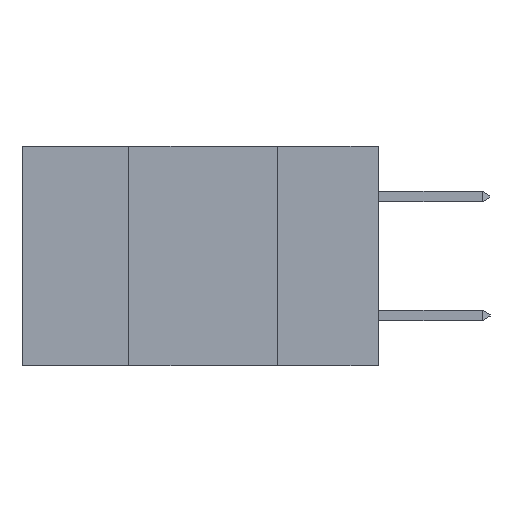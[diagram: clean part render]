
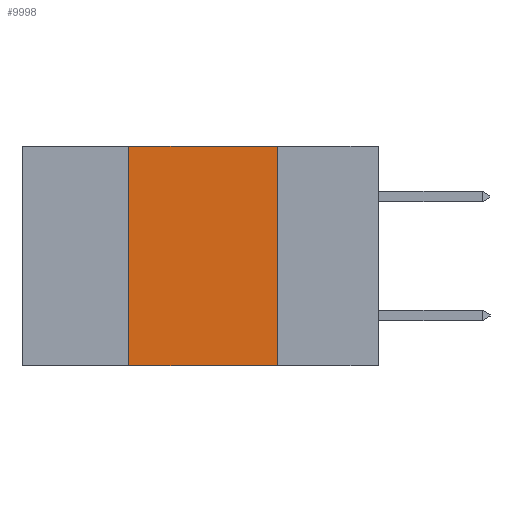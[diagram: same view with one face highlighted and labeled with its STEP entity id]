
A CAD part, left-side view. The second image highlights one B-rep face of the part: STEP entity #9998.
In plain terms, the highlighted planar face has unit normal (-1, 0, 0).
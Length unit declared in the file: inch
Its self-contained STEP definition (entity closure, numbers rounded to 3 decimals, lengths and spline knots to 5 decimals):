
#521 = PLANE ( 'NONE',  #1733 ) ;
#551 = EDGE_CURVE ( 'NONE', #2668, #3006, #5153, .T. ) ;
#586 = CARTESIAN_POINT ( 'NONE',  ( 0., 0.42, -0.37 ) ) ;
#589 = DIRECTION ( 'NONE',  ( 0., -1., 0. ) ) ;
#631 = CARTESIAN_POINT ( 'NONE',  ( 0., 0.6, 0. ) ) ;
#1246 = LINE ( 'NONE', #586, #11676 ) ;
#1620 = DIRECTION ( 'NONE',  ( 0., -1., 0. ) ) ;
#1733 = AXIS2_PLACEMENT_3D ( 'NONE', #4606, #11656, #5645 ) ;
#2446 = LINE ( 'NONE', #10931, #9868 ) ;
#2668 = VERTEX_POINT ( 'NONE', #11022 ) ;
#3006 = VERTEX_POINT ( 'NONE', #3551 ) ;
#3188 = ORIENTED_EDGE ( 'NONE', *, *, #551, .T. ) ;
#3551 = CARTESIAN_POINT ( 'NONE',  ( 0., 0.17, -0.37 ) ) ;
#4606 = CARTESIAN_POINT ( 'NONE',  ( 0., 0.6, 0. ) ) ;
#4994 = CARTESIAN_POINT ( 'NONE',  ( 0., 0.17, 0. ) ) ;
#5034 = VECTOR ( 'NONE', #1620, 39.37008 ) ;
#5153 = LINE ( 'NONE', #8229, #7512 ) ;
#5388 = VERTEX_POINT ( 'NONE', #4994 ) ;
#5645 = DIRECTION ( 'NONE',  ( 0., 0., -1. ) ) ;
#6658 = DIRECTION ( 'NONE',  ( 0., 0., 1. ) ) ;
#7511 = VERTEX_POINT ( 'NONE', #7907 ) ;
#7512 = VECTOR ( 'NONE', #589, 39.37008 ) ;
#7907 = CARTESIAN_POINT ( 'NONE',  ( 0., 0.42, 0. ) ) ;
#8229 = CARTESIAN_POINT ( 'NONE',  ( 0., 0.6, -0.37 ) ) ;
#9337 = EDGE_CURVE ( 'NONE', #2668, #7511, #1246, .T. ) ;
#9868 = VECTOR ( 'NONE', #12939, 39.37008 ) ;
#9998 = ADVANCED_FACE ( 'NONE', ( #10397 ), #521, .F. ) ;
#10266 = ORIENTED_EDGE ( 'NONE', *, *, #12061, .F. ) ;
#10358 = LINE ( 'NONE', #631, #5034 ) ;
#10396 = EDGE_LOOP ( 'NONE', ( #10266, #12310, #12461, #3188 ) ) ;
#10397 = FACE_OUTER_BOUND ( 'NONE', #10396, .T. ) ;
#10931 = CARTESIAN_POINT ( 'NONE',  ( 0., 0.17, -0.37 ) ) ;
#11022 = CARTESIAN_POINT ( 'NONE',  ( 0., 0.42, -0.37 ) ) ;
#11368 = EDGE_CURVE ( 'NONE', #7511, #5388, #10358, .T. ) ;
#11656 = DIRECTION ( 'NONE',  ( 1., 0., 0. ) ) ;
#11676 = VECTOR ( 'NONE', #6658, 39.37008 ) ;
#12061 = EDGE_CURVE ( 'NONE', #5388, #3006, #2446, .T. ) ;
#12310 = ORIENTED_EDGE ( 'NONE', *, *, #11368, .F. ) ;
#12461 = ORIENTED_EDGE ( 'NONE', *, *, #9337, .F. ) ;
#12939 = DIRECTION ( 'NONE',  ( 0., 0., -1. ) ) ;
